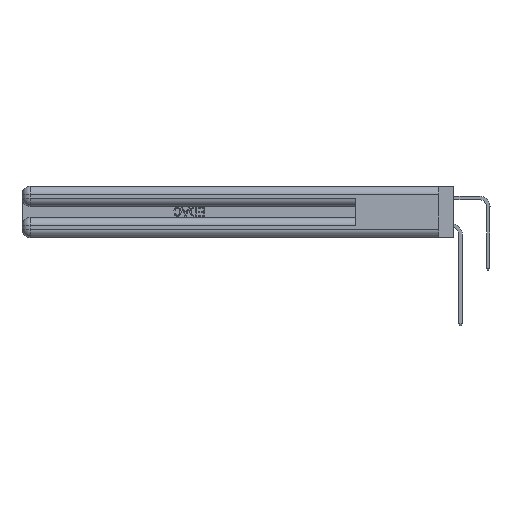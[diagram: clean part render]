
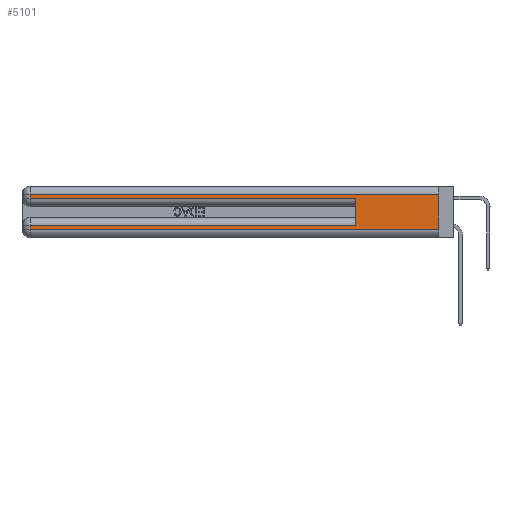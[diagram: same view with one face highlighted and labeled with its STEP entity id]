
A CAD part, left-side view. The second image highlights one B-rep face of the part: STEP entity #5101.
In plain terms, the highlighted planar face has unit normal (-1, 0, 0).
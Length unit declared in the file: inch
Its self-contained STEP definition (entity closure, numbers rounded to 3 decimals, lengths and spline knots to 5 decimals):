
#188 = LINE ( 'NONE', #9368, #18335 ) ;
#437 = LINE ( 'NONE', #39536, #26958 ) ;
#1119 = VERTEX_POINT ( 'NONE', #30770 ) ;
#1242 = CARTESIAN_POINT ( 'NONE',  ( 0., 2.94, 0.285 ) ) ;
#4715 = DIRECTION ( 'NONE',  ( 1., 0., 0. ) ) ;
#5101 = ADVANCED_FACE ( 'NONE', ( #40969 ), #44028, .F. ) ;
#7170 = VERTEX_POINT ( 'NONE', #22266 ) ;
#7222 = VECTOR ( 'NONE', #38343, 39.37008 ) ;
#8155 = ORIENTED_EDGE ( 'NONE', *, *, #32313, .T. ) ;
#8392 = LINE ( 'NONE', #34762, #7222 ) ;
#8968 = LINE ( 'NONE', #40183, #44765 ) ;
#9368 = CARTESIAN_POINT ( 'NONE',  ( 0., 0., 0.285 ) ) ;
#10009 = VERTEX_POINT ( 'NONE', #21025 ) ;
#10546 = VERTEX_POINT ( 'NONE', #20218 ) ;
#10925 = DIRECTION ( 'NONE',  ( 0., 0., -1. ) ) ;
#12581 = CARTESIAN_POINT ( 'NONE',  ( 0., 0.6, 0.085 ) ) ;
#13834 = CARTESIAN_POINT ( 'NONE',  ( 0., 2.94, 0.31 ) ) ;
#14230 = DIRECTION ( 'NONE',  ( 0., 0., 1. ) ) ;
#15504 = VERTEX_POINT ( 'NONE', #13834 ) ;
#15765 = CARTESIAN_POINT ( 'NONE',  ( 0., 0., 0.37 ) ) ;
#16307 = EDGE_CURVE ( 'NONE', #15504, #45424, #437, .T. ) ;
#17174 = CARTESIAN_POINT ( 'NONE',  ( 0., 0., 0.31 ) ) ;
#17713 = VECTOR ( 'NONE', #44875, 39.37008 ) ;
#17759 = LINE ( 'NONE', #42798, #26133 ) ;
#17763 = EDGE_CURVE ( 'NONE', #42161, #1119, #25676, .T. ) ;
#18335 = VECTOR ( 'NONE', #41610, 39.37008 ) ;
#18850 = CARTESIAN_POINT ( 'NONE',  ( 0., 0., 0.085 ) ) ;
#18872 = EDGE_CURVE ( 'NONE', #42161, #7170, #17759, .T. ) ;
#19086 = CARTESIAN_POINT ( 'NONE',  ( 0., 0., 0.37 ) ) ;
#19304 = ORIENTED_EDGE ( 'NONE', *, *, #24742, .T. ) ;
#19324 = DIRECTION ( 'NONE',  ( 0., 0., -1. ) ) ;
#19637 = ORIENTED_EDGE ( 'NONE', *, *, #32584, .T. ) ;
#19973 = LINE ( 'NONE', #41324, #17713 ) ;
#20218 = CARTESIAN_POINT ( 'NONE',  ( 0., 2.94, 0.06 ) ) ;
#21025 = CARTESIAN_POINT ( 'NONE',  ( 0., 0., 0.06 ) ) ;
#22266 = CARTESIAN_POINT ( 'NONE',  ( 0., 0.6, 0.285 ) ) ;
#23009 = EDGE_CURVE ( 'NONE', #1119, #10546, #8392, .T. ) ;
#23728 = ORIENTED_EDGE ( 'NONE', *, *, #16307, .T. ) ;
#24742 = EDGE_CURVE ( 'NONE', #45424, #7170, #188, .T. ) ;
#25676 = LINE ( 'NONE', #18850, #36276 ) ;
#26133 = VECTOR ( 'NONE', #14230, 39.37008 ) ;
#26958 = VECTOR ( 'NONE', #10925, 39.37008 ) ;
#26974 = VECTOR ( 'NONE', #19324, 39.37008 ) ;
#27124 = ORIENTED_EDGE ( 'NONE', *, *, #23009, .T. ) ;
#29845 = DIRECTION ( 'NONE',  ( 0., 0., -1. ) ) ;
#30770 = CARTESIAN_POINT ( 'NONE',  ( 0., 2.94, 0.085 ) ) ;
#31675 = ORIENTED_EDGE ( 'NONE', *, *, #18872, .F. ) ;
#32313 = EDGE_CURVE ( 'NONE', #10546, #10009, #8968, .T. ) ;
#32584 = EDGE_CURVE ( 'NONE', #39593, #15504, #19973, .T. ) ;
#34583 = AXIS2_PLACEMENT_3D ( 'NONE', #19086, #4715, #29845 ) ;
#34762 = CARTESIAN_POINT ( 'NONE',  ( 0., 2.94, 0.37 ) ) ;
#36161 = ORIENTED_EDGE ( 'NONE', *, *, #44753, .F. ) ;
#36276 = VECTOR ( 'NONE', #40215, 39.37008 ) ;
#38343 = DIRECTION ( 'NONE',  ( 0., 0., -1. ) ) ;
#39536 = CARTESIAN_POINT ( 'NONE',  ( 0., 2.94, 0.37 ) ) ;
#39593 = VERTEX_POINT ( 'NONE', #17174 ) ;
#40183 = CARTESIAN_POINT ( 'NONE',  ( 0., 0., 0.06 ) ) ;
#40215 = DIRECTION ( 'NONE',  ( 0., 1., 0. ) ) ;
#40969 = FACE_OUTER_BOUND ( 'NONE', #46399, .T. ) ;
#40981 = ORIENTED_EDGE ( 'NONE', *, *, #17763, .T. ) ;
#41324 = CARTESIAN_POINT ( 'NONE',  ( 0., 0., 0.31 ) ) ;
#41610 = DIRECTION ( 'NONE',  ( 0., -1., 0. ) ) ;
#42161 = VERTEX_POINT ( 'NONE', #12581 ) ;
#42798 = CARTESIAN_POINT ( 'NONE',  ( 0., 0.6, 0.145 ) ) ;
#43627 = DIRECTION ( 'NONE',  ( 0., -1., 0. ) ) ;
#44028 = PLANE ( 'NONE',  #34583 ) ;
#44753 = EDGE_CURVE ( 'NONE', #39593, #10009, #45900, .T. ) ;
#44765 = VECTOR ( 'NONE', #43627, 39.37008 ) ;
#44875 = DIRECTION ( 'NONE',  ( 0., 1., 0. ) ) ;
#45424 = VERTEX_POINT ( 'NONE', #1242 ) ;
#45900 = LINE ( 'NONE', #15765, #26974 ) ;
#46399 = EDGE_LOOP ( 'NONE', ( #36161, #19637, #23728, #19304, #31675, #40981, #27124, #8155 ) ) ;
